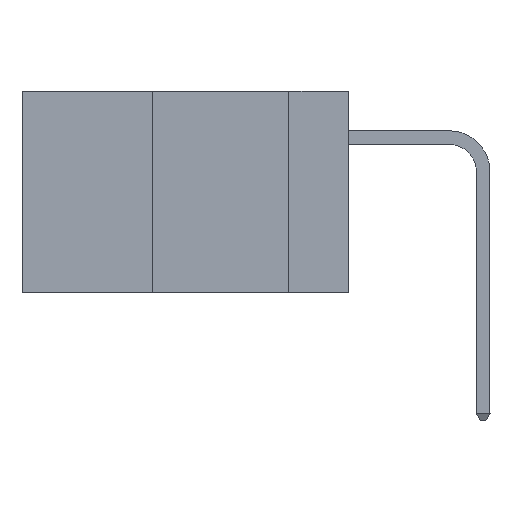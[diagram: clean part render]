
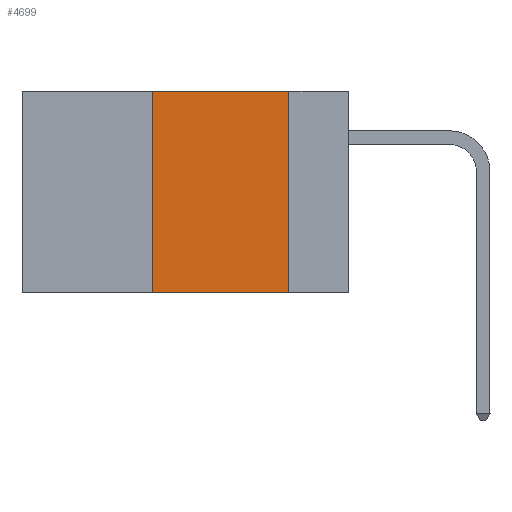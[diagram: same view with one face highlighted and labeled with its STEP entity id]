
A CAD part, left-side view. The second image highlights one B-rep face of the part: STEP entity #4699.
In plain terms, the highlighted planar face has unit normal (-1, 0, 0).
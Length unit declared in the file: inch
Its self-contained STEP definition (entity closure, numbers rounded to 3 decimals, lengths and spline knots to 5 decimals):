
#1447 = CARTESIAN_POINT ( 'NONE',  ( 0., 0.6, 0. ) ) ;
#2610 = FACE_OUTER_BOUND ( 'NONE', #11288, .T. ) ;
#2868 = VECTOR ( 'NONE', #19319, 39.37008 ) ;
#4606 = CARTESIAN_POINT ( 'NONE',  ( 0., 0.36, -0.37 ) ) ;
#4699 = ADVANCED_FACE ( 'NONE', ( #2610 ), #30823, .F. ) ;
#4827 = LINE ( 'NONE', #29500, #26061 ) ;
#5317 = VERTEX_POINT ( 'NONE', #4606 ) ;
#8579 = VERTEX_POINT ( 'NONE', #31137 ) ;
#10678 = ORIENTED_EDGE ( 'NONE', *, *, #18997, .F. ) ;
#11288 = EDGE_LOOP ( 'NONE', ( #10678, #13860, #35608, #16129 ) ) ;
#11722 = CARTESIAN_POINT ( 'NONE',  ( 0., 0.36, 0. ) ) ;
#11878 = DIRECTION ( 'NONE',  ( 0., 0., -1. ) ) ;
#12452 = EDGE_CURVE ( 'NONE', #5317, #40150, #15248, .T. ) ;
#13158 = VERTEX_POINT ( 'NONE', #24303 ) ;
#13860 = ORIENTED_EDGE ( 'NONE', *, *, #39867, .F. ) ;
#15248 = LINE ( 'NONE', #11722, #33449 ) ;
#15414 = CARTESIAN_POINT ( 'NONE',  ( 0., 0.36, 0. ) ) ;
#15996 = LINE ( 'NONE', #1447, #19651 ) ;
#16129 = ORIENTED_EDGE ( 'NONE', *, *, #36235, .T. ) ;
#16500 = LINE ( 'NONE', #16715, #2868 ) ;
#16715 = CARTESIAN_POINT ( 'NONE',  ( 0., 0.6, -0.37 ) ) ;
#18997 = EDGE_CURVE ( 'NONE', #13158, #8579, #4827, .T. ) ;
#19081 = AXIS2_PLACEMENT_3D ( 'NONE', #27513, #37872, #31046 ) ;
#19319 = DIRECTION ( 'NONE',  ( 0., -1., 0. ) ) ;
#19651 = VECTOR ( 'NONE', #26337, 39.37008 ) ;
#24303 = CARTESIAN_POINT ( 'NONE',  ( 0., 0.11, 0. ) ) ;
#26061 = VECTOR ( 'NONE', #11878, 39.37008 ) ;
#26337 = DIRECTION ( 'NONE',  ( 0., -1., 0. ) ) ;
#27513 = CARTESIAN_POINT ( 'NONE',  ( 0., 0.6, 0. ) ) ;
#29500 = CARTESIAN_POINT ( 'NONE',  ( 0., 0.11, 0. ) ) ;
#30823 = PLANE ( 'NONE',  #19081 ) ;
#31046 = DIRECTION ( 'NONE',  ( 0., 0., -1. ) ) ;
#31137 = CARTESIAN_POINT ( 'NONE',  ( 0., 0.11, -0.37 ) ) ;
#33449 = VECTOR ( 'NONE', #33808, 39.37008 ) ;
#33808 = DIRECTION ( 'NONE',  ( 0., 0., 1. ) ) ;
#35608 = ORIENTED_EDGE ( 'NONE', *, *, #12452, .F. ) ;
#36235 = EDGE_CURVE ( 'NONE', #5317, #8579, #16500, .T. ) ;
#37872 = DIRECTION ( 'NONE',  ( 1., 0., 0. ) ) ;
#39867 = EDGE_CURVE ( 'NONE', #40150, #13158, #15996, .T. ) ;
#40150 = VERTEX_POINT ( 'NONE', #15414 ) ;
